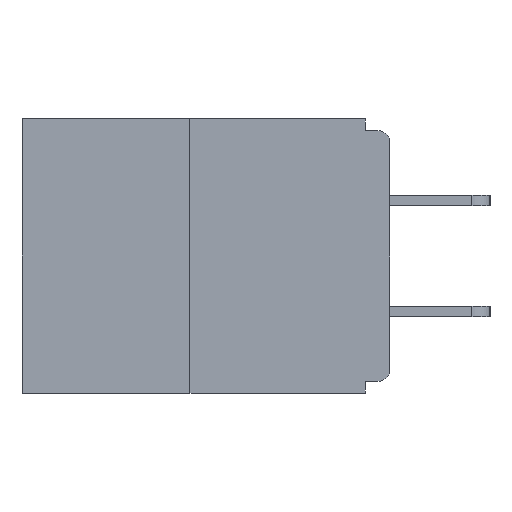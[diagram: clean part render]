
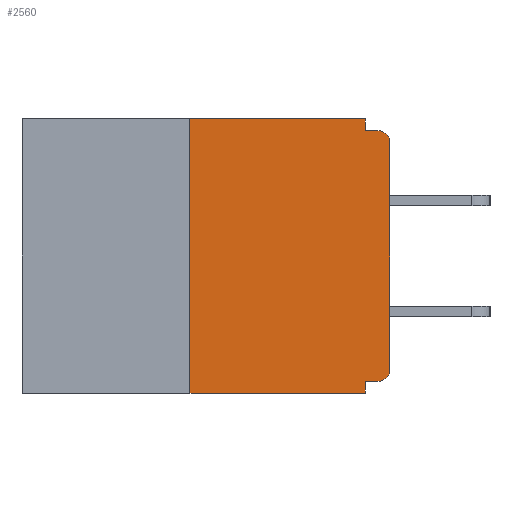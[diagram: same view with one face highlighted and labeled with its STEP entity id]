
A CAD part, left-side view. The second image highlights one B-rep face of the part: STEP entity #2560.
In plain terms, the highlighted planar face has unit normal (-1, 0, 0).
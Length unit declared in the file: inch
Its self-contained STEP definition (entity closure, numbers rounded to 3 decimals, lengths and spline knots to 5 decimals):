
#164 = VECTOR ( 'NONE', #553, 39.37008 ) ;
#259 = DIRECTION ( 'NONE',  ( 0., 0., 1. ) ) ;
#440 = VERTEX_POINT ( 'NONE', #12010 ) ;
#553 = DIRECTION ( 'NONE',  ( 0., 0., 1. ) ) ;
#929 = LINE ( 'NONE', #9191, #21282 ) ;
#1150 = VERTEX_POINT ( 'NONE', #16850 ) ;
#1635 = DIRECTION ( 'NONE',  ( 1., 0., 0. ) ) ;
#1982 = LINE ( 'NONE', #13819, #7403 ) ;
#2217 = EDGE_CURVE ( 'NONE', #10509, #1150, #7928, .T. ) ;
#2560 = ADVANCED_FACE ( 'NONE', ( #5048 ), #18144, .F. ) ;
#2637 = ORIENTED_EDGE ( 'NONE', *, *, #19083, .F. ) ;
#2799 = EDGE_CURVE ( 'NONE', #17237, #20812, #1982, .T. ) ;
#2930 = DIRECTION ( 'NONE',  ( 0., -1., 0. ) ) ;
#3046 = DIRECTION ( 'NONE',  ( -1., 0., 0. ) ) ;
#3092 = ORIENTED_EDGE ( 'NONE', *, *, #13524, .T. ) ;
#3147 = CARTESIAN_POINT ( 'NONE',  ( 0., 0.25, 0. ) ) ;
#3301 = VECTOR ( 'NONE', #6350, 39.37008 ) ;
#3551 = CARTESIAN_POINT ( 'NONE',  ( 0., 0., -0.328 ) ) ;
#3610 = VERTEX_POINT ( 'NONE', #3147 ) ;
#3792 = LINE ( 'NONE', #12903, #21317 ) ;
#4524 = LINE ( 'NONE', #13547, #164 ) ;
#4683 = ORIENTED_EDGE ( 'NONE', *, *, #6825, .T. ) ;
#4894 = DIRECTION ( 'NONE',  ( 0., -1., 0. ) ) ;
#5048 = FACE_OUTER_BOUND ( 'NONE', #11381, .T. ) ;
#5089 = VECTOR ( 'NONE', #4894, 39.37008 ) ;
#5502 = ORIENTED_EDGE ( 'NONE', *, *, #8644, .F. ) ;
#5666 = DIRECTION ( 'NONE',  ( 0., -1., 0. ) ) ;
#5667 = CARTESIAN_POINT ( 'NONE',  ( 0., 0.031, 0. ) ) ;
#5770 = CARTESIAN_POINT ( 'NONE',  ( 0., 0.015, -0.328 ) ) ;
#6238 = ORIENTED_EDGE ( 'NONE', *, *, #17706, .T. ) ;
#6350 = DIRECTION ( 'NONE',  ( 0., 0., -1. ) ) ;
#6825 = EDGE_CURVE ( 'NONE', #13887, #10509, #13541, .T. ) ;
#7340 = ORIENTED_EDGE ( 'NONE', *, *, #19349, .F. ) ;
#7403 = VECTOR ( 'NONE', #15470, 39.37008 ) ;
#7781 = VECTOR ( 'NONE', #259, 39.37008 ) ;
#7821 = CARTESIAN_POINT ( 'NONE',  ( 0., 0.015, -0.03 ) ) ;
#7928 = CIRCLE ( 'NONE', #12132, 0.015 ) ;
#8381 = EDGE_CURVE ( 'NONE', #10624, #1150, #16064, .T. ) ;
#8644 = EDGE_CURVE ( 'NONE', #21283, #10624, #13235, .T. ) ;
#9191 = CARTESIAN_POINT ( 'NONE',  ( 0., 0.46, 0. ) ) ;
#9368 = AXIS2_PLACEMENT_3D ( 'NONE', #17107, #1635, #15270 ) ;
#9959 = CARTESIAN_POINT ( 'NONE',  ( 0., 0., -0.03 ) ) ;
#10509 = VERTEX_POINT ( 'NONE', #9959 ) ;
#10624 = VERTEX_POINT ( 'NONE', #16309 ) ;
#11324 = DIRECTION ( 'NONE',  ( 0., 0., -1. ) ) ;
#11381 = EDGE_LOOP ( 'NONE', ( #7340, #2637, #3092, #20379, #14158, #6238, #4683, #14207, #17389, #5502 ) ) ;
#11521 = LINE ( 'NONE', #3551, #18826 ) ;
#11557 = DIRECTION ( 'NONE',  ( 0., 0., -1. ) ) ;
#12010 = CARTESIAN_POINT ( 'NONE',  ( 0., 0.25, -0.343 ) ) ;
#12132 = AXIS2_PLACEMENT_3D ( 'NONE', #7821, #3046, #11324 ) ;
#12903 = CARTESIAN_POINT ( 'NONE',  ( 0., 0.46, -0.343 ) ) ;
#12989 = CIRCLE ( 'NONE', #16928, 0.015 ) ;
#13147 = CARTESIAN_POINT ( 'NONE',  ( 0., 0.031, 0. ) ) ;
#13235 = LINE ( 'NONE', #13147, #3301 ) ;
#13474 = CARTESIAN_POINT ( 'NONE',  ( 0., 0.015, -0.313 ) ) ;
#13524 = EDGE_CURVE ( 'NONE', #440, #20812, #3792, .T. ) ;
#13541 = LINE ( 'NONE', #16888, #7781 ) ;
#13547 = CARTESIAN_POINT ( 'NONE',  ( 0., 0.25, 0. ) ) ;
#13819 = CARTESIAN_POINT ( 'NONE',  ( 0., 0.031, -0.343 ) ) ;
#13887 = VERTEX_POINT ( 'NONE', #17402 ) ;
#14158 = ORIENTED_EDGE ( 'NONE', *, *, #15914, .F. ) ;
#14207 = ORIENTED_EDGE ( 'NONE', *, *, #2217, .T. ) ;
#14782 = DIRECTION ( 'NONE',  ( -1., 0., 0. ) ) ;
#14827 = CARTESIAN_POINT ( 'NONE',  ( 0., 0.031, -0.343 ) ) ;
#15270 = DIRECTION ( 'NONE',  ( 0., 0., -1. ) ) ;
#15470 = DIRECTION ( 'NONE',  ( 0., 0., -1. ) ) ;
#15914 = EDGE_CURVE ( 'NONE', #21443, #17237, #11521, .T. ) ;
#16064 = LINE ( 'NONE', #20103, #5089 ) ;
#16309 = CARTESIAN_POINT ( 'NONE',  ( 0., 0.031, -0.015 ) ) ;
#16850 = CARTESIAN_POINT ( 'NONE',  ( 0., 0.015, -0.015 ) ) ;
#16888 = CARTESIAN_POINT ( 'NONE',  ( 0., 0., 0. ) ) ;
#16892 = DIRECTION ( 'NONE',  ( 0., 1., 0. ) ) ;
#16928 = AXIS2_PLACEMENT_3D ( 'NONE', #13474, #14782, #11557 ) ;
#17107 = CARTESIAN_POINT ( 'NONE',  ( 0., 0.46, 0. ) ) ;
#17237 = VERTEX_POINT ( 'NONE', #18359 ) ;
#17389 = ORIENTED_EDGE ( 'NONE', *, *, #8381, .F. ) ;
#17402 = CARTESIAN_POINT ( 'NONE',  ( 0., 0., -0.313 ) ) ;
#17706 = EDGE_CURVE ( 'NONE', #21443, #13887, #12989, .T. ) ;
#18144 = PLANE ( 'NONE',  #9368 ) ;
#18359 = CARTESIAN_POINT ( 'NONE',  ( 0., 0.031, -0.328 ) ) ;
#18826 = VECTOR ( 'NONE', #16892, 39.37008 ) ;
#19083 = EDGE_CURVE ( 'NONE', #440, #3610, #4524, .T. ) ;
#19349 = EDGE_CURVE ( 'NONE', #3610, #21283, #929, .T. ) ;
#20103 = CARTESIAN_POINT ( 'NONE',  ( 0., 0., -0.015 ) ) ;
#20379 = ORIENTED_EDGE ( 'NONE', *, *, #2799, .F. ) ;
#20812 = VERTEX_POINT ( 'NONE', #14827 ) ;
#21282 = VECTOR ( 'NONE', #5666, 39.37008 ) ;
#21283 = VERTEX_POINT ( 'NONE', #5667 ) ;
#21317 = VECTOR ( 'NONE', #2930, 39.37008 ) ;
#21443 = VERTEX_POINT ( 'NONE', #5770 ) ;
